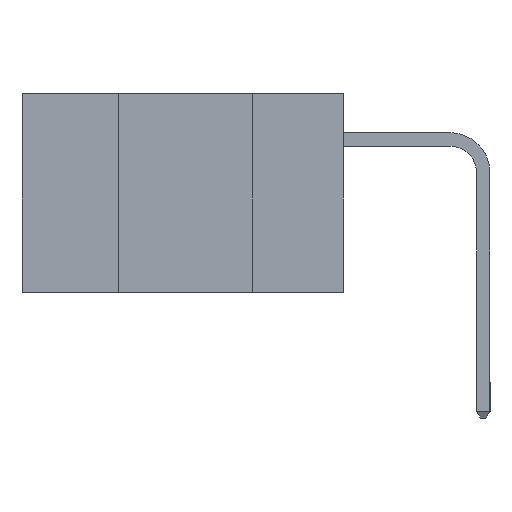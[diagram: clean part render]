
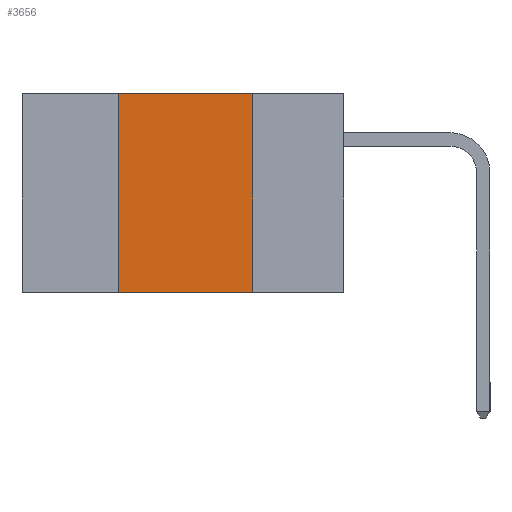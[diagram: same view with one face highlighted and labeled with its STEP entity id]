
A CAD part, left-side view. The second image highlights one B-rep face of the part: STEP entity #3656.
In plain terms, the highlighted planar face has unit normal (-1, 0, 0).
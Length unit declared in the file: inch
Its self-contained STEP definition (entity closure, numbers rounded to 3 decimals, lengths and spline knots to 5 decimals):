
#282 = VERTEX_POINT ( 'NONE', #11815 ) ;
#758 = CARTESIAN_POINT ( 'NONE',  ( 0., 0.6, 0. ) ) ;
#950 = VERTEX_POINT ( 'NONE', #7016 ) ;
#1461 = EDGE_CURVE ( 'NONE', #13019, #950, #1920, .T. ) ;
#1920 = LINE ( 'NONE', #10268, #3171 ) ;
#2036 = DIRECTION ( 'NONE',  ( 0., 0., 1. ) ) ;
#2837 = ORIENTED_EDGE ( 'NONE', *, *, #5548, .F. ) ;
#2865 = LINE ( 'NONE', #2995, #3234 ) ;
#2893 = DIRECTION ( 'NONE',  ( 0., -1., 0. ) ) ;
#2995 = CARTESIAN_POINT ( 'NONE',  ( 0., 0.6, 0. ) ) ;
#3171 = VECTOR ( 'NONE', #2036, 39.37008 ) ;
#3182 = EDGE_LOOP ( 'NONE', ( #5804, #2837, #8980, #10645 ) ) ;
#3234 = VECTOR ( 'NONE', #2893, 39.37008 ) ;
#3392 = EDGE_CURVE ( 'NONE', #13019, #282, #7104, .T. ) ;
#3656 = ADVANCED_FACE ( 'NONE', ( #4572 ), #5217, .F. ) ;
#4572 = FACE_OUTER_BOUND ( 'NONE', #3182, .T. ) ;
#5217 = PLANE ( 'NONE',  #12438 ) ;
#5405 = EDGE_CURVE ( 'NONE', #13607, #282, #10475, .T. ) ;
#5548 = EDGE_CURVE ( 'NONE', #950, #13607, #2865, .T. ) ;
#5804 = ORIENTED_EDGE ( 'NONE', *, *, #5405, .F. ) ;
#6002 = DIRECTION ( 'NONE',  ( 0., -1., 0. ) ) ;
#6290 = CARTESIAN_POINT ( 'NONE',  ( 0., 0.17, 0. ) ) ;
#6319 = DIRECTION ( 'NONE',  ( 1., 0., 0. ) ) ;
#6690 = VECTOR ( 'NONE', #10865, 39.37008 ) ;
#6986 = CARTESIAN_POINT ( 'NONE',  ( 0., 0.6, -0.37 ) ) ;
#7016 = CARTESIAN_POINT ( 'NONE',  ( 0., 0.42, 0. ) ) ;
#7104 = LINE ( 'NONE', #6986, #11083 ) ;
#8839 = CARTESIAN_POINT ( 'NONE',  ( 0., 0.17, 0. ) ) ;
#8980 = ORIENTED_EDGE ( 'NONE', *, *, #1461, .F. ) ;
#10268 = CARTESIAN_POINT ( 'NONE',  ( 0., 0.42, 0. ) ) ;
#10475 = LINE ( 'NONE', #6290, #6690 ) ;
#10645 = ORIENTED_EDGE ( 'NONE', *, *, #3392, .T. ) ;
#10865 = DIRECTION ( 'NONE',  ( 0., 0., -1. ) ) ;
#11083 = VECTOR ( 'NONE', #6002, 39.37008 ) ;
#11102 = DIRECTION ( 'NONE',  ( 0., 0., -1. ) ) ;
#11815 = CARTESIAN_POINT ( 'NONE',  ( 0., 0.17, -0.37 ) ) ;
#12438 = AXIS2_PLACEMENT_3D ( 'NONE', #758, #6319, #11102 ) ;
#13019 = VERTEX_POINT ( 'NONE', #13200 ) ;
#13200 = CARTESIAN_POINT ( 'NONE',  ( 0., 0.42, -0.37 ) ) ;
#13607 = VERTEX_POINT ( 'NONE', #8839 ) ;
